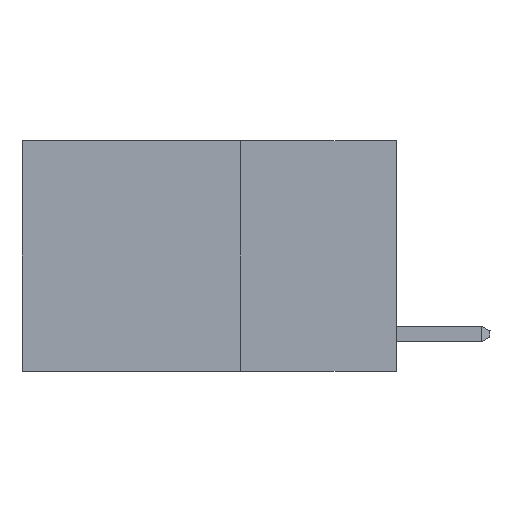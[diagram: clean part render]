
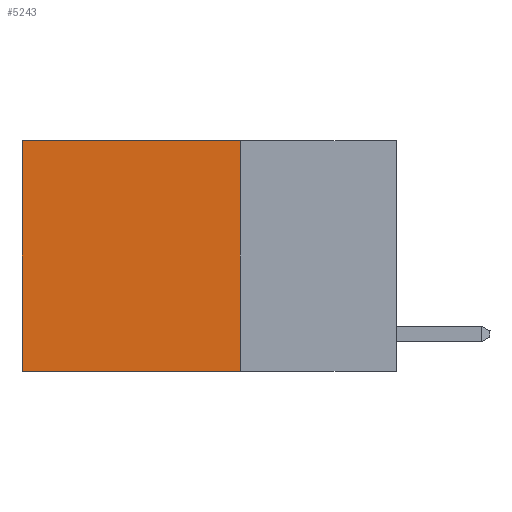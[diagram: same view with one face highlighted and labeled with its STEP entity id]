
A CAD part, left-side view. The second image highlights one B-rep face of the part: STEP entity #5243.
In plain terms, the highlighted planar face has unit normal (-1, 0, 0).
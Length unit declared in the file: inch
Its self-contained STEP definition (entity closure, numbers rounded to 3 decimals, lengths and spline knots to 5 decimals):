
#32 = DIRECTION ( 'NONE',  ( 0., 0., -1. ) ) ;
#79 = VECTOR ( 'NONE', #111, 39.37008 ) ;
#111 = DIRECTION ( 'NONE',  ( 0., 1., 0. ) ) ;
#363 = DIRECTION ( 'NONE',  ( 1., 0., 0. ) ) ;
#2843 = CARTESIAN_POINT ( 'NONE',  ( 0.2625, 0.25, 0. ) ) ;
#4480 = LINE ( 'NONE', #2843, #14249 ) ;
#5243 = ADVANCED_FACE ( 'NONE', ( #22441 ), #12075, .F. ) ;
#6019 = CARTESIAN_POINT ( 'NONE',  ( 0.2625, 0.25, 0. ) ) ;
#6589 = ORIENTED_EDGE ( 'NONE', *, *, #19388, .F. ) ;
#7373 = AXIS2_PLACEMENT_3D ( 'NONE', #23771, #363, #14022 ) ;
#7847 = CARTESIAN_POINT ( 'NONE',  ( 0.2625, 0.6, 0. ) ) ;
#7970 = EDGE_CURVE ( 'NONE', #24260, #23262, #19847, .T. ) ;
#8145 = ORIENTED_EDGE ( 'NONE', *, *, #7970, .T. ) ;
#9897 = CARTESIAN_POINT ( 'NONE',  ( 0.2625, 0.25, -0.37 ) ) ;
#10075 = ORIENTED_EDGE ( 'NONE', *, *, #16374, .F. ) ;
#11247 = CARTESIAN_POINT ( 'NONE',  ( 0.2625, 0.6, -0.37 ) ) ;
#11961 = CARTESIAN_POINT ( 'NONE',  ( 0.2625, 0.6, 0. ) ) ;
#12075 = PLANE ( 'NONE',  #7373 ) ;
#13210 = VERTEX_POINT ( 'NONE', #11247 ) ;
#13365 = EDGE_CURVE ( 'NONE', #23262, #13210, #23786, .T. ) ;
#13465 = ORIENTED_EDGE ( 'NONE', *, *, #13365, .T. ) ;
#13778 = CARTESIAN_POINT ( 'NONE',  ( 0.2625, 0.25, -0.37 ) ) ;
#14022 = DIRECTION ( 'NONE',  ( 0., 0., -1. ) ) ;
#14249 = VECTOR ( 'NONE', #24370, 39.37008 ) ;
#14411 = VERTEX_POINT ( 'NONE', #13778 ) ;
#14793 = CARTESIAN_POINT ( 'NONE',  ( 0.2625, 0.25, 0. ) ) ;
#15166 = EDGE_LOOP ( 'NONE', ( #13465, #10075, #6589, #8145 ) ) ;
#15856 = VECTOR ( 'NONE', #19655, 39.37008 ) ;
#16374 = EDGE_CURVE ( 'NONE', #14411, #13210, #20868, .T. ) ;
#19388 = EDGE_CURVE ( 'NONE', #24260, #14411, #4480, .T. ) ;
#19655 = DIRECTION ( 'NONE',  ( 0., 1., 0. ) ) ;
#19847 = LINE ( 'NONE', #6019, #15856 ) ;
#20868 = LINE ( 'NONE', #9897, #79 ) ;
#22441 = FACE_OUTER_BOUND ( 'NONE', #15166, .T. ) ;
#23178 = VECTOR ( 'NONE', #32, 39.37008 ) ;
#23262 = VERTEX_POINT ( 'NONE', #11961 ) ;
#23771 = CARTESIAN_POINT ( 'NONE',  ( 0.2625, 0.25, 0. ) ) ;
#23786 = LINE ( 'NONE', #7847, #23178 ) ;
#24260 = VERTEX_POINT ( 'NONE', #14793 ) ;
#24370 = DIRECTION ( 'NONE',  ( 0., 0., -1. ) ) ;
